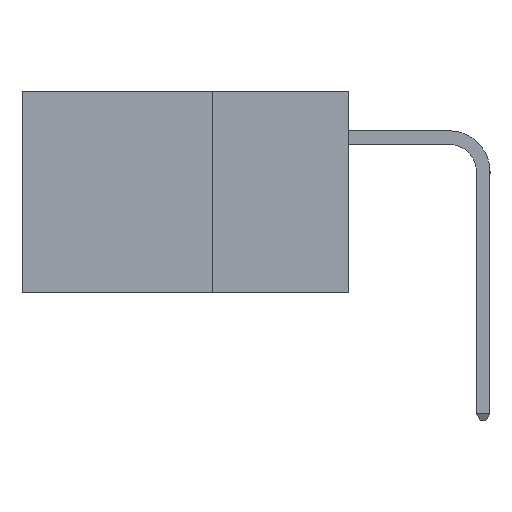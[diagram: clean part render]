
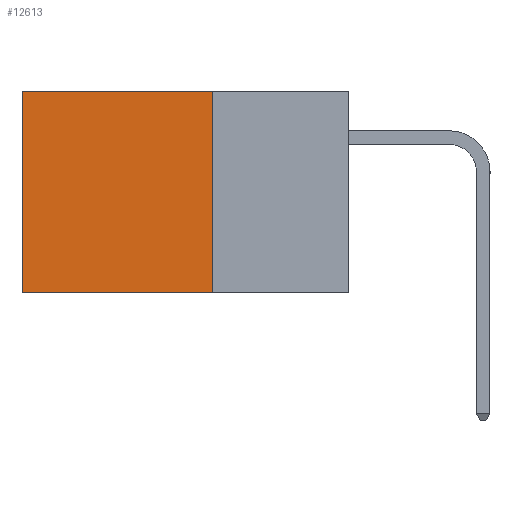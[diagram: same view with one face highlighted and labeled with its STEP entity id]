
A CAD part, left-side view. The second image highlights one B-rep face of the part: STEP entity #12613.
In plain terms, the highlighted planar face has unit normal (-1, 0, 0).
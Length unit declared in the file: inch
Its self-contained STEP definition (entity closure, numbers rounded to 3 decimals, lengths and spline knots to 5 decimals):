
#131 = VECTOR ( 'NONE', #354, 39.37008 ) ;
#132 = PLANE ( 'NONE',  #759 ) ;
#354 = DIRECTION ( 'NONE',  ( 0., 0., -1. ) ) ;
#759 = AXIS2_PLACEMENT_3D ( 'NONE', #7342, #8333, #2250 ) ;
#863 = DIRECTION ( 'NONE',  ( 0., 0., -1. ) ) ;
#1346 = ORIENTED_EDGE ( 'NONE', *, *, #2255, .T. ) ;
#1402 = LINE ( 'NONE', #5210, #4161 ) ;
#1504 = VERTEX_POINT ( 'NONE', #1943 ) ;
#1943 = CARTESIAN_POINT ( 'NONE',  ( 0.2875, 0.6, 0. ) ) ;
#2250 = DIRECTION ( 'NONE',  ( 0., 0., -1. ) ) ;
#2255 = EDGE_CURVE ( 'NONE', #10855, #1504, #1402, .T. ) ;
#2285 = VECTOR ( 'NONE', #5220, 39.37008 ) ;
#2715 = CARTESIAN_POINT ( 'NONE',  ( 0.2875, 0.25, -0.37 ) ) ;
#3280 = EDGE_LOOP ( 'NONE', ( #5204, #4067, #3787, #1346 ) ) ;
#3375 = DIRECTION ( 'NONE',  ( 0., 1., 0. ) ) ;
#3559 = LINE ( 'NONE', #12477, #131 ) ;
#3562 = FACE_OUTER_BOUND ( 'NONE', #3280, .T. ) ;
#3787 = ORIENTED_EDGE ( 'NONE', *, *, #4001, .F. ) ;
#4001 = EDGE_CURVE ( 'NONE', #10855, #6973, #12730, .T. ) ;
#4067 = ORIENTED_EDGE ( 'NONE', *, *, #11851, .F. ) ;
#4161 = VECTOR ( 'NONE', #3375, 39.37008 ) ;
#4755 = VECTOR ( 'NONE', #863, 39.37008 ) ;
#5020 = LINE ( 'NONE', #7235, #2285 ) ;
#5204 = ORIENTED_EDGE ( 'NONE', *, *, #6175, .T. ) ;
#5210 = CARTESIAN_POINT ( 'NONE',  ( 0.2875, 0.25, 0. ) ) ;
#5220 = DIRECTION ( 'NONE',  ( 0., 1., 0. ) ) ;
#6175 = EDGE_CURVE ( 'NONE', #1504, #7359, #3559, .T. ) ;
#6379 = CARTESIAN_POINT ( 'NONE',  ( 0.2875, 0.6, -0.37 ) ) ;
#6973 = VERTEX_POINT ( 'NONE', #2715 ) ;
#7235 = CARTESIAN_POINT ( 'NONE',  ( 0.2875, 0.25, -0.37 ) ) ;
#7342 = CARTESIAN_POINT ( 'NONE',  ( 0.2875, 0.25, 0. ) ) ;
#7359 = VERTEX_POINT ( 'NONE', #6379 ) ;
#8333 = DIRECTION ( 'NONE',  ( 1., 0., 0. ) ) ;
#9033 = CARTESIAN_POINT ( 'NONE',  ( 0.2875, 0.25, 0. ) ) ;
#10855 = VERTEX_POINT ( 'NONE', #11442 ) ;
#11442 = CARTESIAN_POINT ( 'NONE',  ( 0.2875, 0.25, 0. ) ) ;
#11851 = EDGE_CURVE ( 'NONE', #6973, #7359, #5020, .T. ) ;
#12477 = CARTESIAN_POINT ( 'NONE',  ( 0.2875, 0.6, 0. ) ) ;
#12613 = ADVANCED_FACE ( 'NONE', ( #3562 ), #132, .F. ) ;
#12730 = LINE ( 'NONE', #9033, #4755 ) ;
